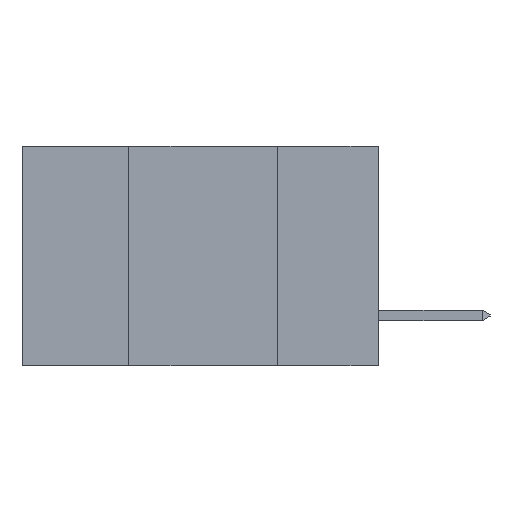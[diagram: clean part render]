
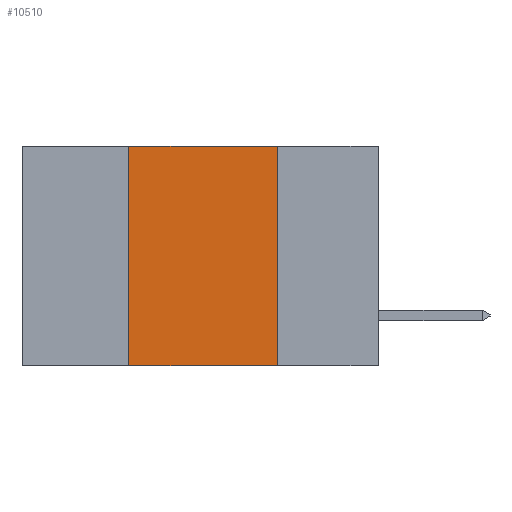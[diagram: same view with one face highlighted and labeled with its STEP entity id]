
A CAD part, left-side view. The second image highlights one B-rep face of the part: STEP entity #10510.
In plain terms, the highlighted planar face has unit normal (-1, 0, 0).
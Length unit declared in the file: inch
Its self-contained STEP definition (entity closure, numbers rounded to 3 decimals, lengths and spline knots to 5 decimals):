
#1296 = PLANE ( 'NONE',  #19226 ) ;
#2676 = ORIENTED_EDGE ( 'NONE', *, *, #11321, .F. ) ;
#3026 = DIRECTION ( 'NONE',  ( 1., 0., 0. ) ) ;
#3147 = DIRECTION ( 'NONE',  ( 0., -1., 0. ) ) ;
#3180 = CARTESIAN_POINT ( 'NONE',  ( 0., 0.6, -0.37 ) ) ;
#3322 = DIRECTION ( 'NONE',  ( 0., -1., 0. ) ) ;
#3392 = CARTESIAN_POINT ( 'NONE',  ( 0., 0.6, 0. ) ) ;
#5987 = VECTOR ( 'NONE', #3147, 39.37008 ) ;
#6002 = VECTOR ( 'NONE', #17484, 39.37008 ) ;
#6241 = LINE ( 'NONE', #17592, #6002 ) ;
#7058 = EDGE_CURVE ( 'NONE', #8258, #8586, #19754, .T. ) ;
#8124 = ORIENTED_EDGE ( 'NONE', *, *, #9737, .F. ) ;
#8220 = CARTESIAN_POINT ( 'NONE',  ( 0., 0.6, 0. ) ) ;
#8258 = VERTEX_POINT ( 'NONE', #18814 ) ;
#8414 = EDGE_CURVE ( 'NONE', #14270, #8586, #6241, .T. ) ;
#8586 = VERTEX_POINT ( 'NONE', #15488 ) ;
#8609 = VECTOR ( 'NONE', #20689, 39.37008 ) ;
#9488 = CARTESIAN_POINT ( 'NONE',  ( 0., 0.42, 0. ) ) ;
#9737 = EDGE_CURVE ( 'NONE', #10274, #14270, #19708, .T. ) ;
#10274 = VERTEX_POINT ( 'NONE', #9488 ) ;
#10510 = ADVANCED_FACE ( 'NONE', ( #21213 ), #1296, .F. ) ;
#10602 = VECTOR ( 'NONE', #3322, 39.37008 ) ;
#11321 = EDGE_CURVE ( 'NONE', #8258, #10274, #22237, .T. ) ;
#13890 = CARTESIAN_POINT ( 'NONE',  ( 0., 0.42, -0.37 ) ) ;
#14270 = VERTEX_POINT ( 'NONE', #16636 ) ;
#14547 = EDGE_LOOP ( 'NONE', ( #18644, #8124, #2676, #18666 ) ) ;
#15189 = DIRECTION ( 'NONE',  ( 0., 0., -1. ) ) ;
#15488 = CARTESIAN_POINT ( 'NONE',  ( 0., 0.17, -0.37 ) ) ;
#16636 = CARTESIAN_POINT ( 'NONE',  ( 0., 0.17, 0. ) ) ;
#17484 = DIRECTION ( 'NONE',  ( 0., 0., -1. ) ) ;
#17592 = CARTESIAN_POINT ( 'NONE',  ( 0., 0.17, -0.37 ) ) ;
#18644 = ORIENTED_EDGE ( 'NONE', *, *, #8414, .F. ) ;
#18666 = ORIENTED_EDGE ( 'NONE', *, *, #7058, .T. ) ;
#18814 = CARTESIAN_POINT ( 'NONE',  ( 0., 0.42, -0.37 ) ) ;
#19226 = AXIS2_PLACEMENT_3D ( 'NONE', #8220, #3026, #15189 ) ;
#19708 = LINE ( 'NONE', #3392, #10602 ) ;
#19754 = LINE ( 'NONE', #3180, #5987 ) ;
#20689 = DIRECTION ( 'NONE',  ( 0., 0., 1. ) ) ;
#21213 = FACE_OUTER_BOUND ( 'NONE', #14547, .T. ) ;
#22237 = LINE ( 'NONE', #13890, #8609 ) ;
